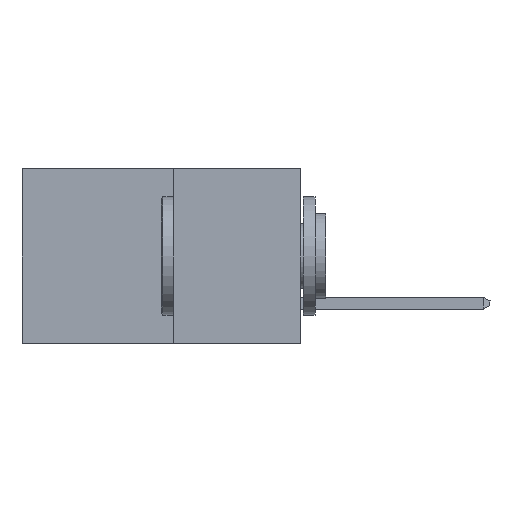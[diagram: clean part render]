
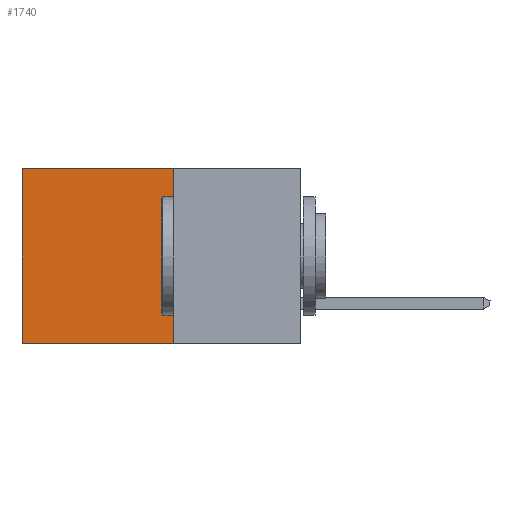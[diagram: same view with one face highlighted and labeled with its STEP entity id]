
A CAD part, left-side view. The second image highlights one B-rep face of the part: STEP entity #1740.
In plain terms, the highlighted planar face has unit normal (-1, 0, 0).
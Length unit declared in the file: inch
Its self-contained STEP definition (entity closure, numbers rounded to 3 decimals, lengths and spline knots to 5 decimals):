
#138 = VERTEX_POINT ( 'NONE', #2106 ) ;
#206 = VERTEX_POINT ( 'NONE', #1071 ) ;
#338 = ORIENTED_EDGE ( 'NONE', *, *, #3847, .F. ) ;
#670 = ORIENTED_EDGE ( 'NONE', *, *, #5395, .T. ) ;
#1071 = CARTESIAN_POINT ( 'NONE',  ( 0.277, 0.59, 0. ) ) ;
#1106 = CARTESIAN_POINT ( 'NONE',  ( 0.277, 0.27, 0. ) ) ;
#1141 = DIRECTION ( 'NONE',  ( 0., 1., 0. ) ) ;
#1257 = VECTOR ( 'NONE', #9822, 39.37008 ) ;
#1295 = CARTESIAN_POINT ( 'NONE',  ( 0.277, 0.27, -0.37 ) ) ;
#1413 = LINE ( 'NONE', #1295, #11851 ) ;
#1740 = ADVANCED_FACE ( 'NONE', ( #9811 ), #2753, .F. ) ;
#1957 = DIRECTION ( 'NONE',  ( 0., 0., -1. ) ) ;
#2106 = CARTESIAN_POINT ( 'NONE',  ( 0.277, 0.27, 0. ) ) ;
#2753 = PLANE ( 'NONE',  #10397 ) ;
#3198 = EDGE_CURVE ( 'NONE', #206, #6822, #3655, .T. ) ;
#3655 = LINE ( 'NONE', #9279, #1257 ) ;
#3847 = EDGE_CURVE ( 'NONE', #10315, #6822, #1413, .T. ) ;
#4103 = CARTESIAN_POINT ( 'NONE',  ( 0.277, 0.27, -0.37 ) ) ;
#5395 = EDGE_CURVE ( 'NONE', #138, #206, #6494, .T. ) ;
#6494 = LINE ( 'NONE', #1106, #11977 ) ;
#6822 = VERTEX_POINT ( 'NONE', #6893 ) ;
#6893 = CARTESIAN_POINT ( 'NONE',  ( 0.277, 0.59, -0.37 ) ) ;
#7068 = CARTESIAN_POINT ( 'NONE',  ( 0.277, 0.27, -0.37 ) ) ;
#7105 = VECTOR ( 'NONE', #1957, 39.37008 ) ;
#8760 = ORIENTED_EDGE ( 'NONE', *, *, #10586, .F. ) ;
#8778 = DIRECTION ( 'NONE',  ( 0., 0., -1. ) ) ;
#9279 = CARTESIAN_POINT ( 'NONE',  ( 0.277, 0.59, -0.37 ) ) ;
#9811 = FACE_OUTER_BOUND ( 'NONE', #10611, .T. ) ;
#9822 = DIRECTION ( 'NONE',  ( 0., 0., -1. ) ) ;
#10315 = VERTEX_POINT ( 'NONE', #10887 ) ;
#10397 = AXIS2_PLACEMENT_3D ( 'NONE', #7068, #12357, #8778 ) ;
#10586 = EDGE_CURVE ( 'NONE', #138, #10315, #12571, .T. ) ;
#10611 = EDGE_LOOP ( 'NONE', ( #11151, #338, #8760, #670 ) ) ;
#10887 = CARTESIAN_POINT ( 'NONE',  ( 0.277, 0.27, -0.37 ) ) ;
#11151 = ORIENTED_EDGE ( 'NONE', *, *, #3198, .T. ) ;
#11249 = DIRECTION ( 'NONE',  ( 0., 1., 0. ) ) ;
#11851 = VECTOR ( 'NONE', #11249, 39.37008 ) ;
#11977 = VECTOR ( 'NONE', #1141, 39.37008 ) ;
#12357 = DIRECTION ( 'NONE',  ( 1., 0., 0. ) ) ;
#12571 = LINE ( 'NONE', #4103, #7105 ) ;
